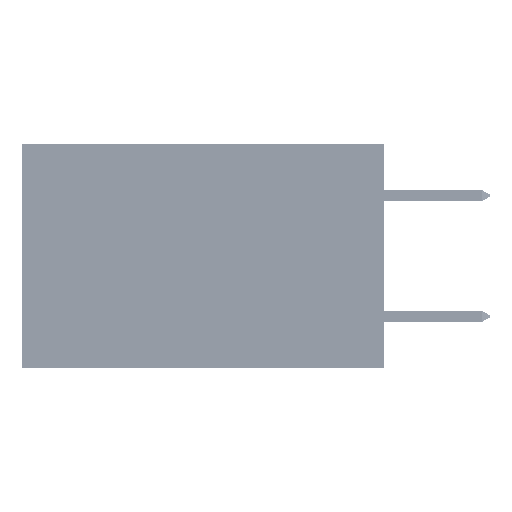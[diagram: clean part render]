
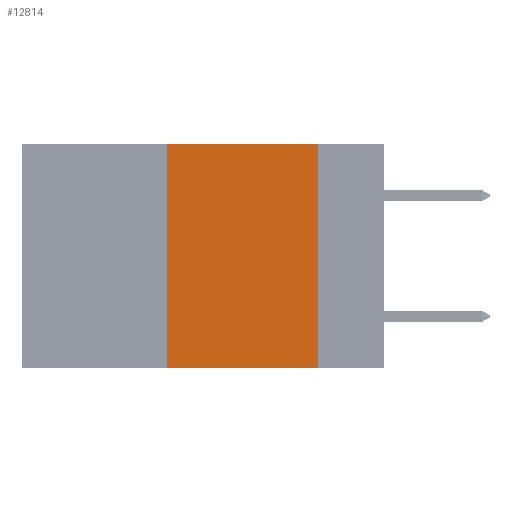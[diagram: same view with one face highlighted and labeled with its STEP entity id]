
A CAD part, left-side view. The second image highlights one B-rep face of the part: STEP entity #12814.
In plain terms, the highlighted planar face has unit normal (-1, 0, 0).
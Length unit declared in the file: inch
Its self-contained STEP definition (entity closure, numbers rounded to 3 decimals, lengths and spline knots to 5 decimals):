
#1421 = CARTESIAN_POINT ( 'NONE',  ( 0., 0.36, -0.37 ) ) ;
#3039 = ORIENTED_EDGE ( 'NONE', *, *, #19607, .F. ) ;
#3879 = VECTOR ( 'NONE', #25010, 39.37008 ) ;
#6753 = VERTEX_POINT ( 'NONE', #23791 ) ;
#7380 = VERTEX_POINT ( 'NONE', #15517 ) ;
#8292 = DIRECTION ( 'NONE',  ( 0., -1., 0. ) ) ;
#9798 = EDGE_CURVE ( 'NONE', #11030, #6753, #28470, .T. ) ;
#10188 = ORIENTED_EDGE ( 'NONE', *, *, #9798, .F. ) ;
#11030 = VERTEX_POINT ( 'NONE', #1421 ) ;
#12667 = EDGE_CURVE ( 'NONE', #11030, #33053, #18870, .T. ) ;
#12814 = ADVANCED_FACE ( 'NONE', ( #46422 ), #38546, .F. ) ;
#13887 = AXIS2_PLACEMENT_3D ( 'NONE', #27221, #34857, #30938 ) ;
#14439 = ORIENTED_EDGE ( 'NONE', *, *, #30207, .F. ) ;
#15517 = CARTESIAN_POINT ( 'NONE',  ( 0., 0.11, 0. ) ) ;
#16251 = CARTESIAN_POINT ( 'NONE',  ( 0., 0.6, 0. ) ) ;
#17470 = VECTOR ( 'NONE', #42594, 39.37008 ) ;
#18304 = CARTESIAN_POINT ( 'NONE',  ( 0., 0.11, -0.37 ) ) ;
#18870 = LINE ( 'NONE', #45704, #24058 ) ;
#19607 = EDGE_CURVE ( 'NONE', #6753, #7380, #34963, .T. ) ;
#20820 = ORIENTED_EDGE ( 'NONE', *, *, #12667, .T. ) ;
#21550 = CARTESIAN_POINT ( 'NONE',  ( 0., 0.36, 0. ) ) ;
#23791 = CARTESIAN_POINT ( 'NONE',  ( 0., 0.36, 0. ) ) ;
#24058 = VECTOR ( 'NONE', #8292, 39.37008 ) ;
#25010 = DIRECTION ( 'NONE',  ( 0., 0., 1. ) ) ;
#27221 = CARTESIAN_POINT ( 'NONE',  ( 0., 0.6, 0. ) ) ;
#28470 = LINE ( 'NONE', #21550, #3879 ) ;
#30207 = EDGE_CURVE ( 'NONE', #7380, #33053, #48004, .T. ) ;
#30938 = DIRECTION ( 'NONE',  ( 0., 0., -1. ) ) ;
#32518 = CARTESIAN_POINT ( 'NONE',  ( 0., 0.11, 0. ) ) ;
#32758 = DIRECTION ( 'NONE',  ( 0., 0., -1. ) ) ;
#33053 = VERTEX_POINT ( 'NONE', #18304 ) ;
#34857 = DIRECTION ( 'NONE',  ( 1., 0., 0. ) ) ;
#34963 = LINE ( 'NONE', #16251, #17470 ) ;
#37436 = EDGE_LOOP ( 'NONE', ( #14439, #3039, #10188, #20820 ) ) ;
#38546 = PLANE ( 'NONE',  #13887 ) ;
#39267 = VECTOR ( 'NONE', #32758, 39.37008 ) ;
#42594 = DIRECTION ( 'NONE',  ( 0., -1., 0. ) ) ;
#45704 = CARTESIAN_POINT ( 'NONE',  ( 0., 0.6, -0.37 ) ) ;
#46422 = FACE_OUTER_BOUND ( 'NONE', #37436, .T. ) ;
#48004 = LINE ( 'NONE', #32518, #39267 ) ;
